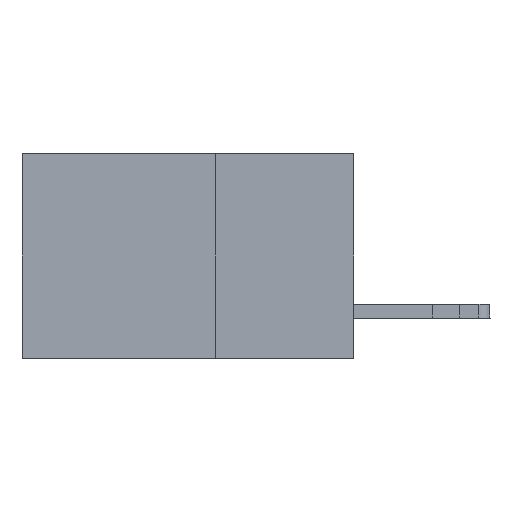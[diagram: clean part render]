
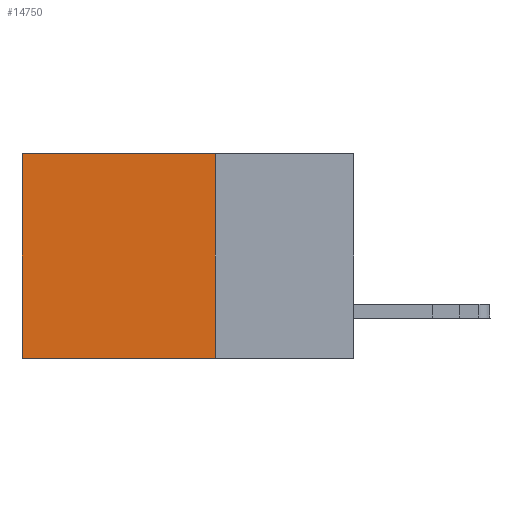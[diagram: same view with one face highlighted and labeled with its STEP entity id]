
A CAD part, left-side view. The second image highlights one B-rep face of the part: STEP entity #14750.
In plain terms, the highlighted planar face has unit normal (-1, 0, 0).
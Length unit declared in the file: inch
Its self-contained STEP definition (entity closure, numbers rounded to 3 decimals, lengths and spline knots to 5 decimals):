
#60 = VERTEX_POINT ( 'NONE', #9743 ) ;
#662 = CARTESIAN_POINT ( 'NONE',  ( 0.2875, 0.6, 0. ) ) ;
#1572 = LINE ( 'NONE', #662, #14089 ) ;
#1826 = CARTESIAN_POINT ( 'NONE',  ( 0.2875, 0.25, -0.37 ) ) ;
#2498 = LINE ( 'NONE', #1826, #13339 ) ;
#3197 = PLANE ( 'NONE',  #11327 ) ;
#3570 = EDGE_LOOP ( 'NONE', ( #6459, #17681, #4025, #11391 ) ) ;
#4025 = ORIENTED_EDGE ( 'NONE', *, *, #16993, .F. ) ;
#4693 = DIRECTION ( 'NONE',  ( 0., 1., 0. ) ) ;
#5224 = EDGE_CURVE ( 'NONE', #60, #5731, #1572, .T. ) ;
#5731 = VERTEX_POINT ( 'NONE', #16828 ) ;
#6067 = DIRECTION ( 'NONE',  ( 0., 0., -1. ) ) ;
#6459 = ORIENTED_EDGE ( 'NONE', *, *, #5224, .T. ) ;
#8169 = DIRECTION ( 'NONE',  ( 0., 0., -1. ) ) ;
#9062 = CARTESIAN_POINT ( 'NONE',  ( 0.2875, 0.25, 0. ) ) ;
#9743 = CARTESIAN_POINT ( 'NONE',  ( 0.2875, 0.6, 0. ) ) ;
#10432 = FACE_OUTER_BOUND ( 'NONE', #3570, .T. ) ;
#10647 = DIRECTION ( 'NONE',  ( 0., 0., -1. ) ) ;
#11327 = AXIS2_PLACEMENT_3D ( 'NONE', #15047, #13351, #10647 ) ;
#11391 = ORIENTED_EDGE ( 'NONE', *, *, #12833, .T. ) ;
#11860 = VECTOR ( 'NONE', #4693, 39.37008 ) ;
#12833 = EDGE_CURVE ( 'NONE', #13055, #60, #16298, .T. ) ;
#13055 = VERTEX_POINT ( 'NONE', #9062 ) ;
#13339 = VECTOR ( 'NONE', #13517, 39.37008 ) ;
#13341 = CARTESIAN_POINT ( 'NONE',  ( 0.2875, 0.25, -0.37 ) ) ;
#13351 = DIRECTION ( 'NONE',  ( 1., 0., 0. ) ) ;
#13517 = DIRECTION ( 'NONE',  ( 0., 1., 0. ) ) ;
#14089 = VECTOR ( 'NONE', #8169, 39.37008 ) ;
#14750 = ADVANCED_FACE ( 'NONE', ( #10432 ), #3197, .F. ) ;
#15047 = CARTESIAN_POINT ( 'NONE',  ( 0.2875, 0.25, 0. ) ) ;
#15104 = CARTESIAN_POINT ( 'NONE',  ( 0.2875, 0.25, 0. ) ) ;
#16298 = LINE ( 'NONE', #15104, #11860 ) ;
#16828 = CARTESIAN_POINT ( 'NONE',  ( 0.2875, 0.6, -0.37 ) ) ;
#16993 = EDGE_CURVE ( 'NONE', #13055, #18813, #17104, .T. ) ;
#17092 = EDGE_CURVE ( 'NONE', #18813, #5731, #2498, .T. ) ;
#17104 = LINE ( 'NONE', #17442, #18711 ) ;
#17442 = CARTESIAN_POINT ( 'NONE',  ( 0.2875, 0.25, 0. ) ) ;
#17681 = ORIENTED_EDGE ( 'NONE', *, *, #17092, .F. ) ;
#18711 = VECTOR ( 'NONE', #6067, 39.37008 ) ;
#18813 = VERTEX_POINT ( 'NONE', #13341 ) ;
